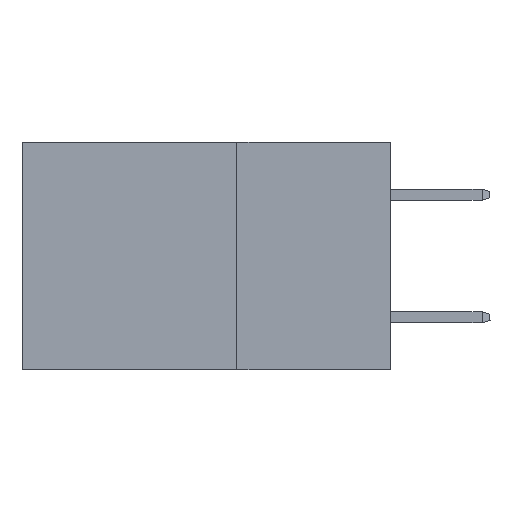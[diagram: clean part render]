
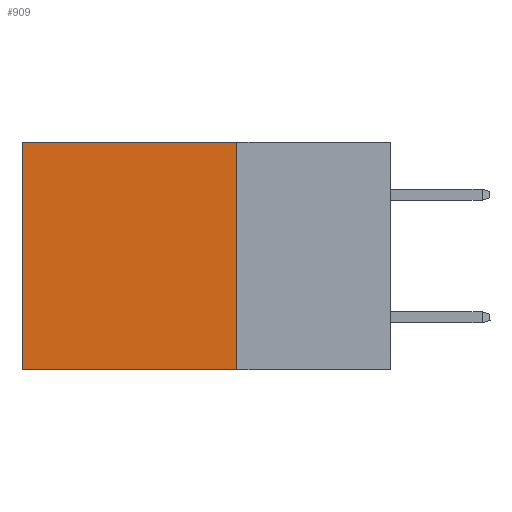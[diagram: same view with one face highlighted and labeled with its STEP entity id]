
A CAD part, left-side view. The second image highlights one B-rep face of the part: STEP entity #909.
In plain terms, the highlighted planar face has unit normal (-1, 0, 0).
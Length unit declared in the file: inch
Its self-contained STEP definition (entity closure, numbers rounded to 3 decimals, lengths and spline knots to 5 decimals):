
#512 = ORIENTED_EDGE ( 'NONE', *, *, #10089, .T. ) ;
#909 = ADVANCED_FACE ( 'NONE', ( #6467 ), #10837, .F. ) ;
#1061 = VECTOR ( 'NONE', #3037, 39.37008 ) ;
#1239 = DIRECTION ( 'NONE',  ( 1., 0., 0. ) ) ;
#1393 = DIRECTION ( 'NONE',  ( 0., 1., 0. ) ) ;
#1483 = ORIENTED_EDGE ( 'NONE', *, *, #9528, .T. ) ;
#2083 = CARTESIAN_POINT ( 'NONE',  ( 0.2875, 0.25, 0. ) ) ;
#2137 = CARTESIAN_POINT ( 'NONE',  ( 0.2875, 0.25, -0.37 ) ) ;
#2688 = CARTESIAN_POINT ( 'NONE',  ( 0.2875, 0.6, 0. ) ) ;
#2702 = ORIENTED_EDGE ( 'NONE', *, *, #4623, .F. ) ;
#3037 = DIRECTION ( 'NONE',  ( 0., 0., -1. ) ) ;
#3481 = DIRECTION ( 'NONE',  ( 0., 0., -1. ) ) ;
#3516 = VECTOR ( 'NONE', #3481, 39.37008 ) ;
#3579 = VECTOR ( 'NONE', #9153, 39.37008 ) ;
#3754 = CARTESIAN_POINT ( 'NONE',  ( 0.2875, 0.25, 0. ) ) ;
#4254 = CARTESIAN_POINT ( 'NONE',  ( 0.2875, 0.6, 0. ) ) ;
#4396 = CARTESIAN_POINT ( 'NONE',  ( 0.2875, 0.25, 0. ) ) ;
#4455 = CARTESIAN_POINT ( 'NONE',  ( 0.2875, 0.25, -0.37 ) ) ;
#4490 = LINE ( 'NONE', #2083, #9030 ) ;
#4623 = EDGE_CURVE ( 'NONE', #5940, #6427, #10023, .T. ) ;
#5911 = CARTESIAN_POINT ( 'NONE',  ( 0.2875, 0.25, 0. ) ) ;
#5940 = VERTEX_POINT ( 'NONE', #4455 ) ;
#6231 = VERTEX_POINT ( 'NONE', #4254 ) ;
#6427 = VERTEX_POINT ( 'NONE', #9149 ) ;
#6467 = FACE_OUTER_BOUND ( 'NONE', #6679, .T. ) ;
#6487 = EDGE_CURVE ( 'NONE', #8467, #5940, #7512, .T. ) ;
#6679 = EDGE_LOOP ( 'NONE', ( #512, #2702, #9935, #1483 ) ) ;
#7155 = AXIS2_PLACEMENT_3D ( 'NONE', #3754, #1239, #9226 ) ;
#7512 = LINE ( 'NONE', #5911, #1061 ) ;
#8467 = VERTEX_POINT ( 'NONE', #4396 ) ;
#9030 = VECTOR ( 'NONE', #1393, 39.37008 ) ;
#9149 = CARTESIAN_POINT ( 'NONE',  ( 0.2875, 0.6, -0.37 ) ) ;
#9153 = DIRECTION ( 'NONE',  ( 0., 1., 0. ) ) ;
#9226 = DIRECTION ( 'NONE',  ( 0., 0., -1. ) ) ;
#9528 = EDGE_CURVE ( 'NONE', #8467, #6231, #4490, .T. ) ;
#9719 = LINE ( 'NONE', #2688, #3516 ) ;
#9935 = ORIENTED_EDGE ( 'NONE', *, *, #6487, .F. ) ;
#10023 = LINE ( 'NONE', #2137, #3579 ) ;
#10089 = EDGE_CURVE ( 'NONE', #6231, #6427, #9719, .T. ) ;
#10837 = PLANE ( 'NONE',  #7155 ) ;
